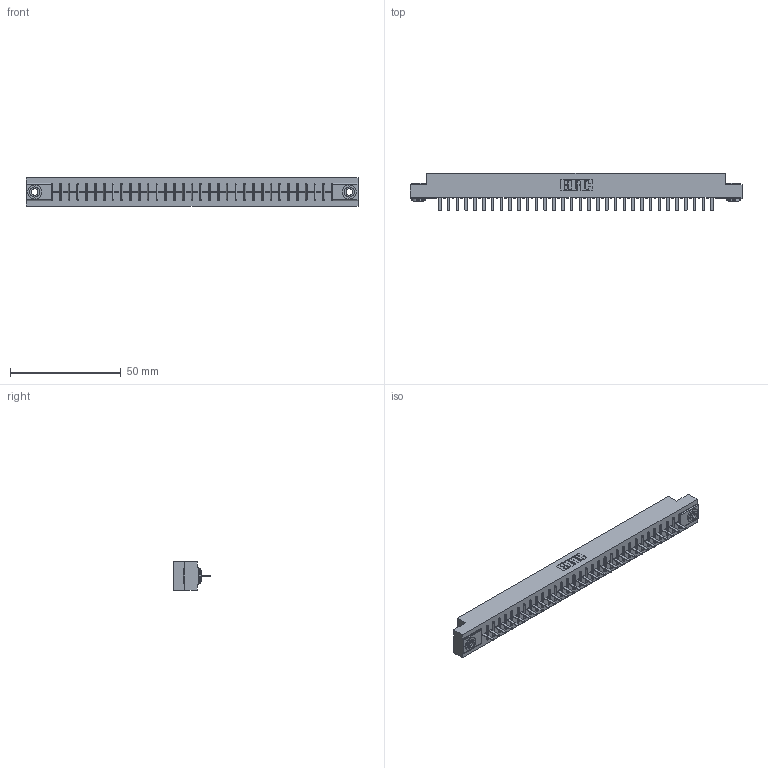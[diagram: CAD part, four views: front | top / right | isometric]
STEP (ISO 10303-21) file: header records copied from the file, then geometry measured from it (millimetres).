
FILE_DESCRIPTION (( 'STEP AP203' ), '1' );
FILE_NAME ('306-032-520-103.STEP', '2019-09-11T22:44:08', ( '' ), ( '' ), 'SwSTEP 2.0', 'SolidWorks 2016', '' );
FILE_SCHEMA (( 'CONFIG_CONTROL_DESIGN' ));
Length unit declared in the file: inch
Products named in the file (4): 306-290-001_120; 345-250-002_345-250-002-102; 306-032-520-103; 306 Part_.156 Dia
Assembly tree (35 placements, depth 2):
  306-032-520-103
    306 Part_.156 Dia
    306-290-001_120  x32
    345-250-002_345-250-002-102  x2
Bounding box: 149.81 x 17.12 x 12.7 mm (x, y, z)
Volume: 16479.5 mm3; surface area: 17078.9 mm2
Topology: 35 solids, 35 shells, 2408 faces, 6732 edges, 4312 vertices
Faces by surface type: plane 1596, cylinder 676, sphere 128, cone 8
Entity records: 32158 total; most frequent: CARTESIAN_POINT 5376, ORIENTED_EDGE 5320, DIRECTION 5316, EDGE_CURVE 2660, LINE 2068, VECTOR 2068, VERTEX_POINT 1684, AXIS2_PLACEMENT_3D 1624
